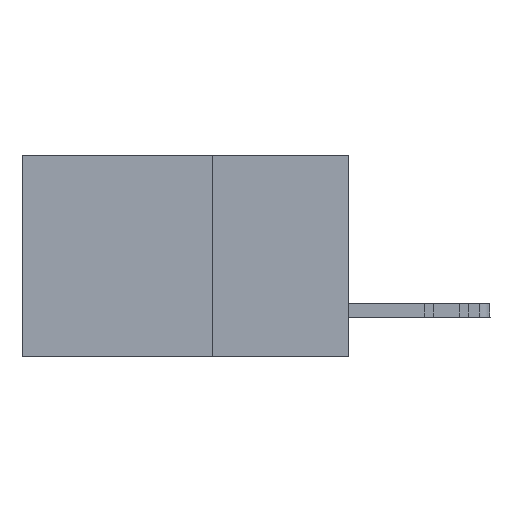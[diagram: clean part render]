
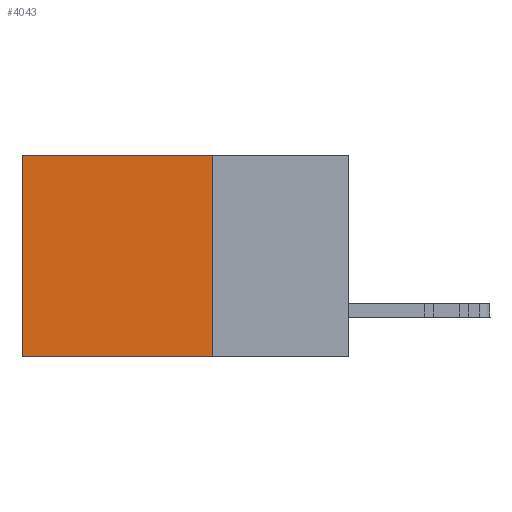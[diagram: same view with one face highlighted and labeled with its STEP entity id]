
A CAD part, left-side view. The second image highlights one B-rep face of the part: STEP entity #4043.
In plain terms, the highlighted planar face has unit normal (-1, 0, 0).
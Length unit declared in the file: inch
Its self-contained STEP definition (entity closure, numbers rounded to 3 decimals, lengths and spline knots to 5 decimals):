
#27 = CARTESIAN_POINT ( 'NONE',  ( 0.298, 0.6, 0. ) ) ;
#423 = VERTEX_POINT ( 'NONE', #27 ) ;
#536 = EDGE_LOOP ( 'NONE', ( #10877, #18957, #22621, #20057 ) ) ;
#1469 = CARTESIAN_POINT ( 'NONE',  ( 0.298, 0.25, -0.37 ) ) ;
#3222 = VECTOR ( 'NONE', #19805, 39.37008 ) ;
#3310 = DIRECTION ( 'NONE',  ( 0., 1., 0. ) ) ;
#4043 = ADVANCED_FACE ( 'NONE', ( #22619 ), #9414, .F. ) ;
#4193 = VECTOR ( 'NONE', #24939, 39.37008 ) ;
#5042 = CARTESIAN_POINT ( 'NONE',  ( 0.298, 0.25, 0. ) ) ;
#6751 = CARTESIAN_POINT ( 'NONE',  ( 0.298, 0.25, 0. ) ) ;
#8100 = LINE ( 'NONE', #23205, #28088 ) ;
#8222 = CARTESIAN_POINT ( 'NONE',  ( 0.298, 0.25, 0. ) ) ;
#9414 = PLANE ( 'NONE',  #13058 ) ;
#10137 = EDGE_CURVE ( 'NONE', #27939, #21652, #8100, .T. ) ;
#10856 = LINE ( 'NONE', #8222, #17109 ) ;
#10877 = ORIENTED_EDGE ( 'NONE', *, *, #25476, .T. ) ;
#13058 = AXIS2_PLACEMENT_3D ( 'NONE', #5042, #16219, #13902 ) ;
#13902 = DIRECTION ( 'NONE',  ( 0., 0., -1. ) ) ;
#15687 = VERTEX_POINT ( 'NONE', #24669 ) ;
#16219 = DIRECTION ( 'NONE',  ( 1., 0., 0. ) ) ;
#16566 = EDGE_CURVE ( 'NONE', #15687, #423, #25666, .T. ) ;
#17109 = VECTOR ( 'NONE', #25794, 39.37008 ) ;
#18957 = ORIENTED_EDGE ( 'NONE', *, *, #10137, .F. ) ;
#19359 = CARTESIAN_POINT ( 'NONE',  ( 0.298, 0.6, -0.37 ) ) ;
#19805 = DIRECTION ( 'NONE',  ( 0., 1., 0. ) ) ;
#20057 = ORIENTED_EDGE ( 'NONE', *, *, #16566, .T. ) ;
#21652 = VERTEX_POINT ( 'NONE', #19359 ) ;
#22616 = CARTESIAN_POINT ( 'NONE',  ( 0.298, 0.6, 0. ) ) ;
#22619 = FACE_OUTER_BOUND ( 'NONE', #536, .T. ) ;
#22621 = ORIENTED_EDGE ( 'NONE', *, *, #22898, .F. ) ;
#22898 = EDGE_CURVE ( 'NONE', #15687, #27939, #10856, .T. ) ;
#23205 = CARTESIAN_POINT ( 'NONE',  ( 0.298, 0.25, -0.37 ) ) ;
#24669 = CARTESIAN_POINT ( 'NONE',  ( 0.298, 0.25, 0. ) ) ;
#24939 = DIRECTION ( 'NONE',  ( 0., 0., -1. ) ) ;
#25476 = EDGE_CURVE ( 'NONE', #423, #21652, #26978, .T. ) ;
#25666 = LINE ( 'NONE', #6751, #3222 ) ;
#25794 = DIRECTION ( 'NONE',  ( 0., 0., -1. ) ) ;
#26978 = LINE ( 'NONE', #22616, #4193 ) ;
#27939 = VERTEX_POINT ( 'NONE', #1469 ) ;
#28088 = VECTOR ( 'NONE', #3310, 39.37008 ) ;
